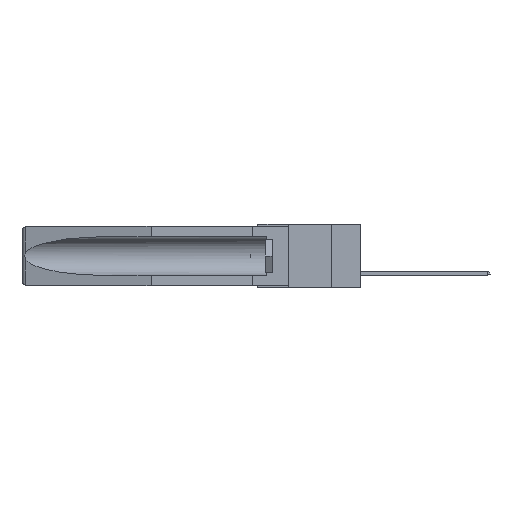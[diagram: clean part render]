
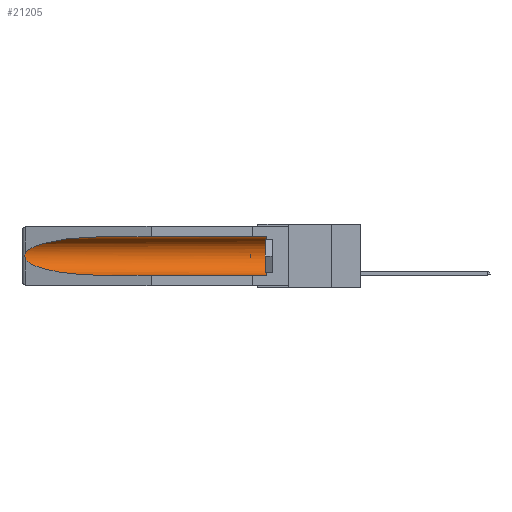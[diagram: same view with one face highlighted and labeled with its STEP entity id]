
A CAD part, left-side view. The second image highlights one B-rep face of the part: STEP entity #21205.
In plain terms, the highlighted cylindrical face has radius 2.857 mm (diameter 5.715 mm), a partial arc.
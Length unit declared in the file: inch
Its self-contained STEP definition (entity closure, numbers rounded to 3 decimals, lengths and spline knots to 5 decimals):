
#61 = CARTESIAN_POINT ( 'NONE',  ( 0.2675, 1.53308, -0.16763 ) ) ;
#197 = EDGE_CURVE ( 'NONE', #27334, #11969, #6901, .T. ) ;
#1075 = EDGE_CURVE ( 'NONE', #14526, #11969, #20567, .T. ) ;
#1629 = ORIENTED_EDGE ( 'NONE', *, *, #29510, .T. ) ;
#2342 = CARTESIAN_POINT ( 'NONE',  ( 0.155, -0.30754, -0.284 ) ) ;
#2729 = CARTESIAN_POINT ( 'NONE',  ( 0.26654, 1.53092, -0.15636 ) ) ;
#3674 = CARTESIAN_POINT ( 'NONE',  ( 0.25451, 1.48313, -0.09465 ) ) ;
#4994 = CARTESIAN_POINT ( 'NONE',  ( 0.155, 0.126, -0.284 ) ) ;
#6274 = LINE ( 'NONE', #15938, #24192 ) ;
#6616 = VERTEX_POINT ( 'NONE', #31699 ) ;
#6901 = LINE ( 'NONE', #2342, #23585 ) ;
#8163 = CARTESIAN_POINT ( 'NONE',  ( 0.26537, 1.52718, -0.19328 ) ) ;
#8445 = DIRECTION ( 'NONE',  ( 0., 1., 0. ) ) ;
#10711 = CARTESIAN_POINT ( 'NONE',  ( 0.2673, 1.53269, -0.17917 ) ) ;
#10943 = AXIS2_PLACEMENT_3D ( 'NONE', #22473, #17187, #14621 ) ;
#11357 = CYLINDRICAL_SURFACE ( 'NONE', #10943, 0.1125 ) ;
#11606 = ORIENTED_EDGE ( 'NONE', *, *, #25706, .T. ) ;
#11969 = VERTEX_POINT ( 'NONE', #15681 ) ;
#12935 = CARTESIAN_POINT ( 'NONE',  ( 0.21114, 1.30732, -0.284 ) ) ;
#13052 = CARTESIAN_POINT ( 'NONE',  ( 0.2673, 1.5327, -0.16383 ) ) ;
#13288 = CARTESIAN_POINT ( 'NONE',  ( 0.26597, 1.52961, -0.15275 ) ) ;
#13973 = CARTESIAN_POINT ( 'NONE',  ( 0.155, 0.126, -0.059 ) ) ;
#14413 = VERTEX_POINT ( 'NONE', #26139 ) ;
#14461 = CARTESIAN_POINT ( 'NONE',  ( 0.155, 0.126, -0.1715 ) ) ;
#14526 = VERTEX_POINT ( 'NONE', #27297 ) ;
#14574 = CARTESIAN_POINT ( 'NONE',  ( 0.26537, 1.52718, -0.14972 ) ) ;
#14621 = DIRECTION ( 'NONE',  ( 0., 0., 1. ) ) ;
#15008 = VERTEX_POINT ( 'NONE', #13973 ) ;
#15530 = FACE_OUTER_BOUND ( 'NONE', #24664, .T. ) ;
#15681 = CARTESIAN_POINT ( 'NONE',  ( 0.155, 1.07973, -0.284 ) ) ;
#15700 = CARTESIAN_POINT ( 'NONE',  ( 0.26597, 1.5296, -0.19026 ) ) ;
#15938 = CARTESIAN_POINT ( 'NONE',  ( 0.155, -0.30754, -0.059 ) ) ;
#16835 = ORIENTED_EDGE ( 'NONE', *, *, #22593, .T. ) ;
#16910 = CARTESIAN_POINT ( 'NONE',  ( 0.21114, 1.30732, -0.059 ) ) ;
#17187 = DIRECTION ( 'NONE',  ( 0., 1., 0. ) ) ;
#17607 = CIRCLE ( 'NONE', #33153, 0.1125 ) ;
#18854 =( BOUNDED_CURVE ( )  B_SPLINE_CURVE ( 3, ( #22184, #16910, #3674, #14574 ),
 .UNSPECIFIED., .F., .F. ) 
 B_SPLINE_CURVE_WITH_KNOTS ( ( 4, 4 ),
 ( 4.71239, 6.08839 ),
 .UNSPECIFIED. ) 
 CURVE ( )  GEOMETRIC_REPRESENTATION_ITEM ( )  RATIONAL_B_SPLINE_CURVE ( ( 1., 0.848, 0.848, 1. ) ) 
 REPRESENTATION_ITEM ( '' )  );
#19276 = DIRECTION ( 'NONE',  ( 0., -1., 0. ) ) ;
#19326 = ORIENTED_EDGE ( 'NONE', *, *, #1075, .T. ) ;
#19890 = EDGE_CURVE ( 'NONE', #14413, #6616, #18854, .T. ) ;
#20567 =( BOUNDED_CURVE ( )  B_SPLINE_CURVE ( 3, ( #26341, #28905, #12935, #31316 ),
 .UNSPECIFIED., .F., .T. ) 
 B_SPLINE_CURVE_WITH_KNOTS ( ( 4, 4 ),
 ( 0.1948, 1.5708 ),
 .UNSPECIFIED. ) 
 CURVE ( )  GEOMETRIC_REPRESENTATION_ITEM ( )  RATIONAL_B_SPLINE_CURVE ( ( 1., 0.848, 0.848, 1. ) ) 
 REPRESENTATION_ITEM ( '' )  );
#20992 = B_SPLINE_CURVE_WITH_KNOTS ( 'NONE', 3,
 ( #26917, #13288, #2729, #13052, #61, #21337, #10711, #34338, #15700, #8163 ),
 .UNSPECIFIED., .F., .F.,
 ( 4, 2, 2, 2, 4 ),
 ( 0., 0.00029, 0.00058, 0.00087, 0.00117 ),
 .UNSPECIFIED. ) ;
#21205 = ADVANCED_FACE ( 'NONE', ( #15530 ), #11357, .F. ) ;
#21337 = CARTESIAN_POINT ( 'NONE',  ( 0.2675, 1.53308, -0.17534 ) ) ;
#22093 = DIRECTION ( 'NONE',  ( 0., 0., 1. ) ) ;
#22184 = CARTESIAN_POINT ( 'NONE',  ( 0.155, 1.07973, -0.059 ) ) ;
#22473 = CARTESIAN_POINT ( 'NONE',  ( 0.155, -0.30754, -0.1715 ) ) ;
#22593 = EDGE_CURVE ( 'NONE', #15008, #14413, #6274, .T. ) ;
#23585 = VECTOR ( 'NONE', #8445, 39.37008 ) ;
#24192 = VECTOR ( 'NONE', #26452, 39.37008 ) ;
#24664 = EDGE_LOOP ( 'NONE', ( #31252, #11606, #19326, #32251, #1629, #16835 ) ) ;
#25706 = EDGE_CURVE ( 'NONE', #6616, #14526, #20992, .T. ) ;
#26139 = CARTESIAN_POINT ( 'NONE',  ( 0.155, 1.07973, -0.059 ) ) ;
#26341 = CARTESIAN_POINT ( 'NONE',  ( 0.26537, 1.52718, -0.19328 ) ) ;
#26452 = DIRECTION ( 'NONE',  ( 0., 1., 0. ) ) ;
#26917 = CARTESIAN_POINT ( 'NONE',  ( 0.26537, 1.52718, -0.14972 ) ) ;
#27297 = CARTESIAN_POINT ( 'NONE',  ( 0.26537, 1.52718, -0.19328 ) ) ;
#27334 = VERTEX_POINT ( 'NONE', #4994 ) ;
#28905 = CARTESIAN_POINT ( 'NONE',  ( 0.25451, 1.48313, -0.24835 ) ) ;
#29510 = EDGE_CURVE ( 'NONE', #27334, #15008, #17607, .T. ) ;
#31252 = ORIENTED_EDGE ( 'NONE', *, *, #19890, .T. ) ;
#31316 = CARTESIAN_POINT ( 'NONE',  ( 0.155, 1.07973, -0.284 ) ) ;
#31699 = CARTESIAN_POINT ( 'NONE',  ( 0.26537, 1.52718, -0.14972 ) ) ;
#32251 = ORIENTED_EDGE ( 'NONE', *, *, #197, .F. ) ;
#33153 = AXIS2_PLACEMENT_3D ( 'NONE', #14461, #19276, #22093 ) ;
#34338 = CARTESIAN_POINT ( 'NONE',  ( 0.26655, 1.53094, -0.18657 ) ) ;
